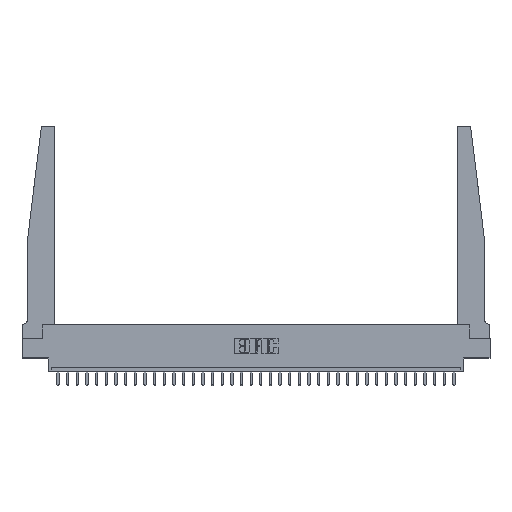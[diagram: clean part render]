
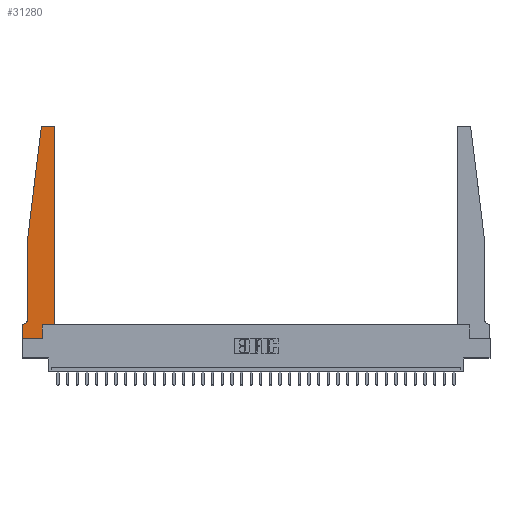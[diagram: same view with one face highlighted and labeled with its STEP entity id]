
A CAD part, top view. The second image highlights one B-rep face of the part: STEP entity #31280.
In plain terms, the highlighted planar face has unit normal (0, 0, 1).
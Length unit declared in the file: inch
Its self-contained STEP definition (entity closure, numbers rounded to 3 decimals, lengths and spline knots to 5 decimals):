
#96 = CARTESIAN_POINT ( 'NONE',  ( 0.25, 2.75, 0.37 ) ) ;
#477 = DIRECTION ( 'NONE',  ( -1., 0., 0. ) ) ;
#1641 = DIRECTION ( 'NONE',  ( 1., 0., 0. ) ) ;
#1999 = ORIENTED_EDGE ( 'NONE', *, *, #6168, .T. ) ;
#2238 = CARTESIAN_POINT ( 'NONE',  ( 0.065, 0.1875, 0.37 ) ) ;
#2852 = ORIENTED_EDGE ( 'NONE', *, *, #12036, .T. ) ;
#2855 = CARTESIAN_POINT ( 'NONE',  ( 0.015, 0.2375, 0.37 ) ) ;
#3031 = VERTEX_POINT ( 'NONE', #20433 ) ;
#3226 = VERTEX_POINT ( 'NONE', #22001 ) ;
#3956 = EDGE_CURVE ( 'NONE', #5130, #8987, #17304, .T. ) ;
#4054 = CARTESIAN_POINT ( 'NONE',  ( 0.065, 1.25, 0.37 ) ) ;
#4620 = LINE ( 'NONE', #2238, #5724 ) ;
#4632 = LINE ( 'NONE', #16918, #6328 ) ;
#5130 = VERTEX_POINT ( 'NONE', #20832 ) ;
#5273 = CARTESIAN_POINT ( 'NONE',  ( 0.065, 0.2375, 0.37 ) ) ;
#5537 = AXIS2_PLACEMENT_3D ( 'NONE', #25994, #13897, #1641 ) ;
#5724 = VECTOR ( 'NONE', #31418, 39.37008 ) ;
#5731 = CARTESIAN_POINT ( 'NONE',  ( 0., 0.1875, 0.37 ) ) ;
#5852 = CARTESIAN_POINT ( 'NONE',  ( 0.065, 1.25, 0.37 ) ) ;
#6167 = EDGE_CURVE ( 'NONE', #8987, #28778, #20802, .T. ) ;
#6168 = EDGE_CURVE ( 'NONE', #17698, #21196, #18681, .T. ) ;
#6328 = VECTOR ( 'NONE', #14669, 39.37008 ) ;
#6445 = ORIENTED_EDGE ( 'NONE', *, *, #19462, .T. ) ;
#6528 = ORIENTED_EDGE ( 'NONE', *, *, #3956, .T. ) ;
#6855 = LINE ( 'NONE', #28245, #22536 ) ;
#6972 = CARTESIAN_POINT ( 'NONE',  ( 0., 0.1875, 0.37 ) ) ;
#7154 = ORIENTED_EDGE ( 'NONE', *, *, #12828, .T. ) ;
#7512 = VECTOR ( 'NONE', #8927, 39.37008 ) ;
#8469 = CARTESIAN_POINT ( 'NONE',  ( 0., 0., 0.37 ) ) ;
#8927 = DIRECTION ( 'NONE',  ( 1., 0., 0. ) ) ;
#8987 = VERTEX_POINT ( 'NONE', #11508 ) ;
#9224 = CIRCLE ( 'NONE', #16387, 0.05 ) ;
#9509 = EDGE_CURVE ( 'NONE', #3226, #30761, #24052, .T. ) ;
#10443 = AXIS2_PLACEMENT_3D ( 'NONE', #6972, #14312, #16567 ) ;
#10576 = CARTESIAN_POINT ( 'NONE',  ( 0.2605, 0.18, 0.37 ) ) ;
#10621 = DIRECTION ( 'NONE',  ( -0.122, -0.992, 0. ) ) ;
#11508 = CARTESIAN_POINT ( 'NONE',  ( 0.27653, 2.75, 0.37 ) ) ;
#11977 = DIRECTION ( 'NONE',  ( 0., 0., -1. ) ) ;
#11985 = ORIENTED_EDGE ( 'NONE', *, *, #6167, .T. ) ;
#12036 = EDGE_CURVE ( 'NONE', #30761, #16395, #21056, .T. ) ;
#12330 = EDGE_LOOP ( 'NONE', ( #6528, #11985, #20939, #7154, #24211, #28233, #1999, #16600, #24592, #2852, #6445, #15137 ) ) ;
#12828 = EDGE_CURVE ( 'NONE', #24950, #19562, #13764, .T. ) ;
#13764 = LINE ( 'NONE', #4054, #17757 ) ;
#13897 = DIRECTION ( 'NONE',  ( 0., 0., 1. ) ) ;
#14001 = FACE_OUTER_BOUND ( 'NONE', #12330, .T. ) ;
#14145 = CARTESIAN_POINT ( 'NONE',  ( 0.24675, 2.72367, 0.37 ) ) ;
#14171 = CARTESIAN_POINT ( 'NONE',  ( 0.2605, 0.18, 0.37 ) ) ;
#14312 = DIRECTION ( 'NONE',  ( 0., 0., 1. ) ) ;
#14669 = DIRECTION ( 'NONE',  ( 1., 0., 0. ) ) ;
#15137 = ORIENTED_EDGE ( 'NONE', *, *, #29331, .T. ) ;
#16131 = DIRECTION ( 'NONE',  ( 0., -1., 0. ) ) ;
#16387 = AXIS2_PLACEMENT_3D ( 'NONE', #2855, #11977, #477 ) ;
#16395 = VERTEX_POINT ( 'NONE', #24831 ) ;
#16567 = DIRECTION ( 'NONE',  ( 1., 0., 0. ) ) ;
#16600 = ORIENTED_EDGE ( 'NONE', *, *, #28485, .T. ) ;
#16615 = CARTESIAN_POINT ( 'NONE',  ( 0., 0., 0.37 ) ) ;
#16918 = CARTESIAN_POINT ( 'NONE',  ( 0., 0., 0.37 ) ) ;
#17094 = VECTOR ( 'NONE', #21984, 39.37008 ) ;
#17145 = CARTESIAN_POINT ( 'NONE',  ( 0.395, 2.72, 0.37 ) ) ;
#17300 = DIRECTION ( 'NONE',  ( 0., 0., 1. ) ) ;
#17304 = LINE ( 'NONE', #96, #28083 ) ;
#17698 = VERTEX_POINT ( 'NONE', #5731 ) ;
#17757 = VECTOR ( 'NONE', #20932, 39.37008 ) ;
#18681 = LINE ( 'NONE', #8469, #25360 ) ;
#18705 = EDGE_CURVE ( 'NONE', #23472, #17698, #4620, .T. ) ;
#18933 = EDGE_CURVE ( 'NONE', #28778, #24950, #29937, .T. ) ;
#19462 = EDGE_CURVE ( 'NONE', #16395, #3031, #6855, .T. ) ;
#19562 = VERTEX_POINT ( 'NONE', #5273 ) ;
#19593 = CARTESIAN_POINT ( 'NONE',  ( 0.015, 0.1875, 0.37 ) ) ;
#20433 = CARTESIAN_POINT ( 'NONE',  ( 0.425, 2.72, 0.37 ) ) ;
#20802 = CIRCLE ( 'NONE', #5537, 0.03 ) ;
#20832 = CARTESIAN_POINT ( 'NONE',  ( 0.395, 2.75, 0.37 ) ) ;
#20932 = DIRECTION ( 'NONE',  ( 0., -1., 0. ) ) ;
#20939 = ORIENTED_EDGE ( 'NONE', *, *, #18933, .T. ) ;
#21056 = LINE ( 'NONE', #30802, #7512 ) ;
#21148 = AXIS2_PLACEMENT_3D ( 'NONE', #17145, #17300, #24448 ) ;
#21196 = VERTEX_POINT ( 'NONE', #16615 ) ;
#21984 = DIRECTION ( 'NONE',  ( 0., 1., 0. ) ) ;
#22001 = CARTESIAN_POINT ( 'NONE',  ( 0.2605, 0., 0.37 ) ) ;
#22536 = VECTOR ( 'NONE', #25989, 39.37008 ) ;
#23472 = VERTEX_POINT ( 'NONE', #19593 ) ;
#24052 = LINE ( 'NONE', #14171, #17094 ) ;
#24211 = ORIENTED_EDGE ( 'NONE', *, *, #24822, .T. ) ;
#24448 = DIRECTION ( 'NONE',  ( 1., 0., 0. ) ) ;
#24592 = ORIENTED_EDGE ( 'NONE', *, *, #9509, .T. ) ;
#24822 = EDGE_CURVE ( 'NONE', #19562, #23472, #9224, .T. ) ;
#24831 = CARTESIAN_POINT ( 'NONE',  ( 0.425, 0.18, 0.37 ) ) ;
#24950 = VERTEX_POINT ( 'NONE', #25146 ) ;
#25146 = CARTESIAN_POINT ( 'NONE',  ( 0.065, 1.25, 0.37 ) ) ;
#25360 = VECTOR ( 'NONE', #16131, 39.37008 ) ;
#25989 = DIRECTION ( 'NONE',  ( 0., 1., 0. ) ) ;
#25994 = CARTESIAN_POINT ( 'NONE',  ( 0.27653, 2.72, 0.37 ) ) ;
#28083 = VECTOR ( 'NONE', #29115, 39.37008 ) ;
#28212 = PLANE ( 'NONE',  #10443 ) ;
#28233 = ORIENTED_EDGE ( 'NONE', *, *, #18705, .T. ) ;
#28245 = CARTESIAN_POINT ( 'NONE',  ( 0.425, 0.18, 0.37 ) ) ;
#28485 = EDGE_CURVE ( 'NONE', #21196, #3226, #4632, .T. ) ;
#28778 = VERTEX_POINT ( 'NONE', #14145 ) ;
#29115 = DIRECTION ( 'NONE',  ( -1., 0., 0. ) ) ;
#29163 = VECTOR ( 'NONE', #10621, 39.37008 ) ;
#29331 = EDGE_CURVE ( 'NONE', #3031, #5130, #30817, .T. ) ;
#29937 = LINE ( 'NONE', #5852, #29163 ) ;
#30761 = VERTEX_POINT ( 'NONE', #10576 ) ;
#30802 = CARTESIAN_POINT ( 'NONE',  ( 0.425, 0.18, 0.37 ) ) ;
#30817 = CIRCLE ( 'NONE', #21148, 0.03 ) ;
#31280 = ADVANCED_FACE ( 'NONE', ( #14001 ), #28212, .T. ) ;
#31418 = DIRECTION ( 'NONE',  ( -1., 0., 0. ) ) ;
